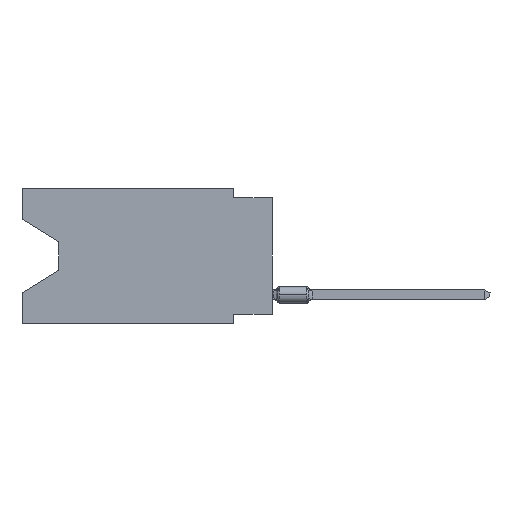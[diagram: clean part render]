
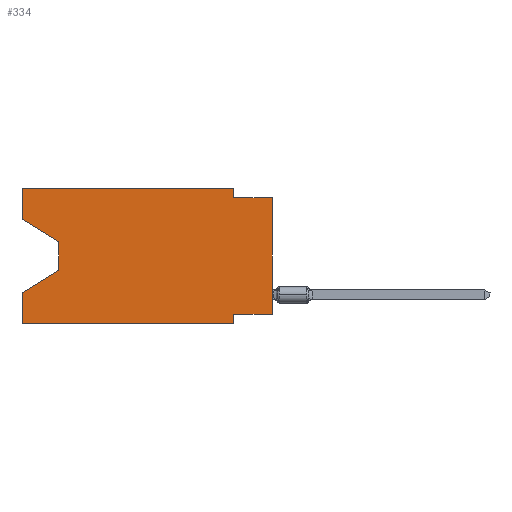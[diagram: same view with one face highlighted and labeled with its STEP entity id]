
A CAD part, left-side view. The second image highlights one B-rep face of the part: STEP entity #334.
In plain terms, the highlighted planar face has unit normal (-1, 0, 0).
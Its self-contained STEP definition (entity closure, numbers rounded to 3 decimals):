
#334 = ADVANCED_FACE ( 'NONE', ( #26700 ), #37374, .F. ) ;
#385 = CARTESIAN_POINT ( 'NONE',  ( 0., 2.54, 0. ) ) ;
#1202 = CARTESIAN_POINT ( 'NONE',  ( 0., 16.383, 0. ) ) ;
#1380 = VECTOR ( 'NONE', #16245, 1000. ) ;
#2083 = LINE ( 'NONE', #27524, #22224 ) ;
#2563 = VERTEX_POINT ( 'NONE', #39156 ) ;
#2613 = DIRECTION ( 'NONE',  ( 0., -0.855, -0.519 ) ) ;
#2909 = VERTEX_POINT ( 'NONE', #25546 ) ;
#3229 = EDGE_CURVE ( 'NONE', #20812, #16201, #26772, .T. ) ;
#3795 = DIRECTION ( 'NONE',  ( 0., 0., -1. ) ) ;
#4303 = ORIENTED_EDGE ( 'NONE', *, *, #26157, .T. ) ;
#5133 = VECTOR ( 'NONE', #22479, 1000. ) ;
#6097 = CARTESIAN_POINT ( 'NONE',  ( 0., 16.383, -8.89 ) ) ;
#6420 = CARTESIAN_POINT ( 'NONE',  ( 0., 2.54, -0.635 ) ) ;
#6573 = VECTOR ( 'NONE', #35908, 1000. ) ;
#6794 = ORIENTED_EDGE ( 'NONE', *, *, #31217, .F. ) ;
#7377 = VECTOR ( 'NONE', #15006, 1000. ) ;
#7413 = CARTESIAN_POINT ( 'NONE',  ( 0., 2.54, -8.89 ) ) ;
#7487 = ORIENTED_EDGE ( 'NONE', *, *, #15263, .F. ) ;
#8623 = ORIENTED_EDGE ( 'NONE', *, *, #13448, .T. ) ;
#9924 = VECTOR ( 'NONE', #19708, 1000. ) ;
#10105 = CARTESIAN_POINT ( 'NONE',  ( 0., 16.383, 0. ) ) ;
#11201 = DIRECTION ( 'NONE',  ( 0., -1., 0. ) ) ;
#12012 = EDGE_CURVE ( 'NONE', #23274, #2563, #24863, .T. ) ;
#13448 = EDGE_CURVE ( 'NONE', #33624, #2909, #2083, .T. ) ;
#13669 = CARTESIAN_POINT ( 'NONE',  ( 0., 13.97, -5.385 ) ) ;
#13947 = EDGE_CURVE ( 'NONE', #30386, #14098, #35125, .T. ) ;
#14046 = ORIENTED_EDGE ( 'NONE', *, *, #23522, .F. ) ;
#14098 = VERTEX_POINT ( 'NONE', #7413 ) ;
#14673 = EDGE_CURVE ( 'NONE', #19638, #33624, #21107, .T. ) ;
#15006 = DIRECTION ( 'NONE',  ( 0., 0., 1. ) ) ;
#15225 = CARTESIAN_POINT ( 'NONE',  ( 0., 16.383, 0. ) ) ;
#15263 = EDGE_CURVE ( 'NONE', #35810, #20827, #29572, .T. ) ;
#15319 = CARTESIAN_POINT ( 'NONE',  ( 0., 0., -0.635 ) ) ;
#16146 = ORIENTED_EDGE ( 'NONE', *, *, #29451, .T. ) ;
#16201 = VERTEX_POINT ( 'NONE', #15319 ) ;
#16245 = DIRECTION ( 'NONE',  ( 0., -1., 0. ) ) ;
#16261 = VECTOR ( 'NONE', #23400, 1000. ) ;
#16632 = LINE ( 'NONE', #1202, #6573 ) ;
#16927 = CARTESIAN_POINT ( 'NONE',  ( 0., 16.383, 0. ) ) ;
#17104 = CARTESIAN_POINT ( 'NONE',  ( 0., 16.383, -2.038 ) ) ;
#17285 = CARTESIAN_POINT ( 'NONE',  ( 0., 0., -8.255 ) ) ;
#17915 = ORIENTED_EDGE ( 'NONE', *, *, #29782, .F. ) ;
#18023 = ORIENTED_EDGE ( 'NONE', *, *, #14673, .T. ) ;
#18669 = LINE ( 'NONE', #28095, #7377 ) ;
#18808 = CARTESIAN_POINT ( 'NONE',  ( 0., 0., -8.255 ) ) ;
#19638 = VERTEX_POINT ( 'NONE', #17104 ) ;
#19708 = DIRECTION ( 'NONE',  ( 0., 0., -1. ) ) ;
#19829 = LINE ( 'NONE', #13669, #5133 ) ;
#20812 = VERTEX_POINT ( 'NONE', #6420 ) ;
#20827 = VERTEX_POINT ( 'NONE', #33106 ) ;
#21077 = VECTOR ( 'NONE', #2613, 1000. ) ;
#21107 = LINE ( 'NONE', #30930, #21077 ) ;
#21354 = AXIS2_PLACEMENT_3D ( 'NONE', #15225, #25218, #21553 ) ;
#21553 = DIRECTION ( 'NONE',  ( 0., 0., -1. ) ) ;
#22049 = ORIENTED_EDGE ( 'NONE', *, *, #3229, .F. ) ;
#22126 = VERTEX_POINT ( 'NONE', #31615 ) ;
#22224 = VECTOR ( 'NONE', #33493, 1000. ) ;
#22479 = DIRECTION ( 'NONE',  ( 0., 0.855, -0.519 ) ) ;
#23274 = VERTEX_POINT ( 'NONE', #16927 ) ;
#23400 = DIRECTION ( 'NONE',  ( 0., 1., 0. ) ) ;
#23522 = EDGE_CURVE ( 'NONE', #30386, #22126, #16632, .T. ) ;
#24260 = VECTOR ( 'NONE', #3795, 1000. ) ;
#24602 = ORIENTED_EDGE ( 'NONE', *, *, #12012, .F. ) ;
#24639 = EDGE_CURVE ( 'NONE', #2563, #20812, #34496, .T. ) ;
#24863 = LINE ( 'NONE', #10105, #1380 ) ;
#25218 = DIRECTION ( 'NONE',  ( 1., 0., 0. ) ) ;
#25546 = CARTESIAN_POINT ( 'NONE',  ( 0., 13.97, -5.385 ) ) ;
#26063 = LINE ( 'NONE', #35539, #39897 ) ;
#26157 = EDGE_CURVE ( 'NONE', #35810, #16201, #18669, .T. ) ;
#26700 = FACE_OUTER_BOUND ( 'NONE', #36839, .T. ) ;
#26772 = LINE ( 'NONE', #39322, #35236 ) ;
#27524 = CARTESIAN_POINT ( 'NONE',  ( 0., 13.97, -3.505 ) ) ;
#28095 = CARTESIAN_POINT ( 'NONE',  ( 0., 0., 0. ) ) ;
#28955 = DIRECTION ( 'NONE',  ( 0., -1., 0. ) ) ;
#29159 = CARTESIAN_POINT ( 'NONE',  ( 0., 16.383, -8.89 ) ) ;
#29451 = EDGE_CURVE ( 'NONE', #2909, #22126, #19829, .T. ) ;
#29572 = LINE ( 'NONE', #17285, #16261 ) ;
#29782 = EDGE_CURVE ( 'NONE', #19638, #23274, #26063, .T. ) ;
#30386 = VERTEX_POINT ( 'NONE', #6097 ) ;
#30930 = CARTESIAN_POINT ( 'NONE',  ( 0., 16.383, -2.038 ) ) ;
#31217 = EDGE_CURVE ( 'NONE', #20827, #14098, #35203, .T. ) ;
#31240 = CARTESIAN_POINT ( 'NONE',  ( 0., 13.97, -3.505 ) ) ;
#31615 = CARTESIAN_POINT ( 'NONE',  ( 0., 16.383, -6.852 ) ) ;
#31900 = CARTESIAN_POINT ( 'NONE',  ( 0., 2.54, -8.89 ) ) ;
#32075 = VECTOR ( 'NONE', #28955, 1000. ) ;
#33106 = CARTESIAN_POINT ( 'NONE',  ( 0., 2.54, -8.255 ) ) ;
#33493 = DIRECTION ( 'NONE',  ( 0., 0., -1. ) ) ;
#33624 = VERTEX_POINT ( 'NONE', #31240 ) ;
#34275 = ORIENTED_EDGE ( 'NONE', *, *, #24639, .F. ) ;
#34496 = LINE ( 'NONE', #385, #9924 ) ;
#35125 = LINE ( 'NONE', #29159, #32075 ) ;
#35203 = LINE ( 'NONE', #31900, #24260 ) ;
#35236 = VECTOR ( 'NONE', #11201, 1000. ) ;
#35539 = CARTESIAN_POINT ( 'NONE',  ( 0., 16.383, 0. ) ) ;
#35810 = VERTEX_POINT ( 'NONE', #18808 ) ;
#35908 = DIRECTION ( 'NONE',  ( 0., 0., 1. ) ) ;
#35933 = DIRECTION ( 'NONE',  ( 0., 0., 1. ) ) ;
#36839 = EDGE_LOOP ( 'NONE', ( #18023, #8623, #16146, #14046, #37468, #6794, #7487, #4303, #22049, #34275, #24602, #17915 ) ) ;
#37374 = PLANE ( 'NONE',  #21354 ) ;
#37468 = ORIENTED_EDGE ( 'NONE', *, *, #13947, .T. ) ;
#39156 = CARTESIAN_POINT ( 'NONE',  ( 0., 2.54, 0. ) ) ;
#39322 = CARTESIAN_POINT ( 'NONE',  ( 0., 0., -0.635 ) ) ;
#39897 = VECTOR ( 'NONE', #35933, 1000. ) ;
